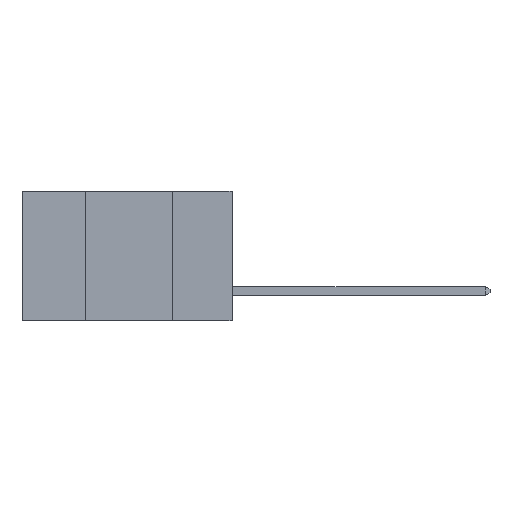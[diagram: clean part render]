
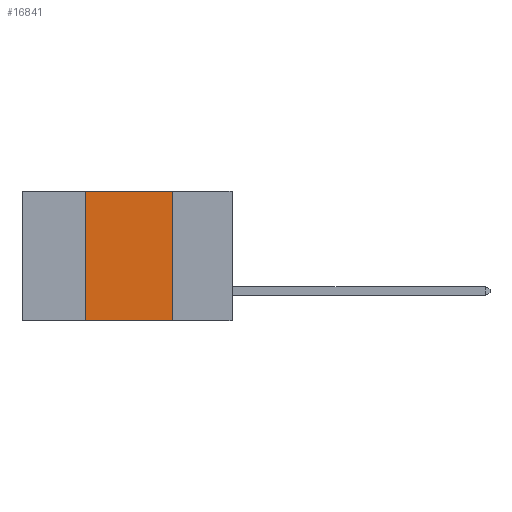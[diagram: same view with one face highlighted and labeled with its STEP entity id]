
A CAD part, left-side view. The second image highlights one B-rep face of the part: STEP entity #16841.
In plain terms, the highlighted planar face has unit normal (-1, 0, 0).
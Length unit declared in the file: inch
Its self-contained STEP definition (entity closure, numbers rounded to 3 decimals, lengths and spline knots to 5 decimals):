
#1193 = VECTOR ( 'NONE', #16232, 39.37008 ) ;
#1430 = ORIENTED_EDGE ( 'NONE', *, *, #1595, .F. ) ;
#1595 = EDGE_CURVE ( 'NONE', #17299, #19710, #11397, .T. ) ;
#1713 = LINE ( 'NONE', #6712, #1193 ) ;
#1890 = DIRECTION ( 'NONE',  ( 0., 0., 1. ) ) ;
#1938 = DIRECTION ( 'NONE',  ( 1., 0., 0. ) ) ;
#2080 = EDGE_LOOP ( 'NONE', ( #1430, #15595, #3085, #5798 ) ) ;
#2597 = CARTESIAN_POINT ( 'NONE',  ( 0., 0.6, 0. ) ) ;
#3085 = ORIENTED_EDGE ( 'NONE', *, *, #16208, .F. ) ;
#3268 = CARTESIAN_POINT ( 'NONE',  ( 0., 0.17, 0. ) ) ;
#3398 = EDGE_CURVE ( 'NONE', #4566, #17299, #4150, .T. ) ;
#4150 = LINE ( 'NONE', #2597, #8570 ) ;
#4386 = DIRECTION ( 'NONE',  ( 0., -1., 0. ) ) ;
#4566 = VERTEX_POINT ( 'NONE', #7095 ) ;
#5798 = ORIENTED_EDGE ( 'NONE', *, *, #11329, .T. ) ;
#6162 = LINE ( 'NONE', #8664, #14214 ) ;
#6449 = CARTESIAN_POINT ( 'NONE',  ( 0., 0.42, -0.37 ) ) ;
#6712 = CARTESIAN_POINT ( 'NONE',  ( 0., 0.6, -0.37 ) ) ;
#7095 = CARTESIAN_POINT ( 'NONE',  ( 0., 0.42, 0. ) ) ;
#7123 = VECTOR ( 'NONE', #11506, 39.37008 ) ;
#8570 = VECTOR ( 'NONE', #4386, 39.37008 ) ;
#8664 = CARTESIAN_POINT ( 'NONE',  ( 0., 0.42, 0. ) ) ;
#8704 = PLANE ( 'NONE',  #11892 ) ;
#11329 = EDGE_CURVE ( 'NONE', #14190, #19710, #1713, .T. ) ;
#11397 = LINE ( 'NONE', #20744, #7123 ) ;
#11506 = DIRECTION ( 'NONE',  ( 0., 0., -1. ) ) ;
#11892 = AXIS2_PLACEMENT_3D ( 'NONE', #11907, #1938, #13534 ) ;
#11907 = CARTESIAN_POINT ( 'NONE',  ( 0., 0.6, 0. ) ) ;
#11939 = CARTESIAN_POINT ( 'NONE',  ( 0., 0.17, -0.37 ) ) ;
#13534 = DIRECTION ( 'NONE',  ( 0., 0., -1. ) ) ;
#14190 = VERTEX_POINT ( 'NONE', #6449 ) ;
#14214 = VECTOR ( 'NONE', #1890, 39.37008 ) ;
#15595 = ORIENTED_EDGE ( 'NONE', *, *, #3398, .F. ) ;
#16208 = EDGE_CURVE ( 'NONE', #14190, #4566, #6162, .T. ) ;
#16232 = DIRECTION ( 'NONE',  ( 0., -1., 0. ) ) ;
#16841 = ADVANCED_FACE ( 'NONE', ( #19961 ), #8704, .F. ) ;
#17299 = VERTEX_POINT ( 'NONE', #3268 ) ;
#19710 = VERTEX_POINT ( 'NONE', #11939 ) ;
#19961 = FACE_OUTER_BOUND ( 'NONE', #2080, .T. ) ;
#20744 = CARTESIAN_POINT ( 'NONE',  ( 0., 0.17, 0. ) ) ;
